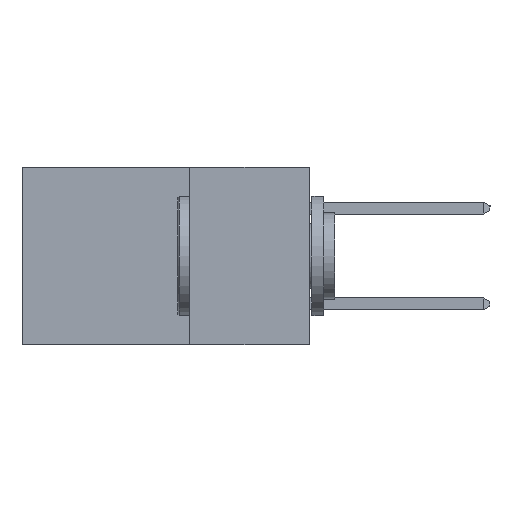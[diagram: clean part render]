
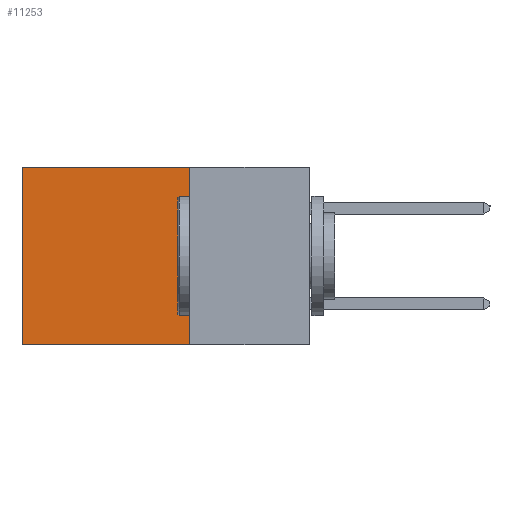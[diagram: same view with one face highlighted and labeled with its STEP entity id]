
A CAD part, left-side view. The second image highlights one B-rep face of the part: STEP entity #11253.
In plain terms, the highlighted planar face has unit normal (-1, 0, 0).
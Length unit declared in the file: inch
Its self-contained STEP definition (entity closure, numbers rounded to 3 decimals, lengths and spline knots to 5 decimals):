
#400 = CARTESIAN_POINT ( 'NONE',  ( 0.2875, 0.25, -0.37 ) ) ;
#543 = EDGE_CURVE ( 'NONE', #21170, #3944, #23759, .T. ) ;
#1645 = DIRECTION ( 'NONE',  ( 0., 0., -1. ) ) ;
#1817 = VECTOR ( 'NONE', #15721, 39.37008 ) ;
#2220 = VECTOR ( 'NONE', #1645, 39.37008 ) ;
#2248 = LINE ( 'NONE', #12837, #2220 ) ;
#3517 = ORIENTED_EDGE ( 'NONE', *, *, #543, .T. ) ;
#3944 = VERTEX_POINT ( 'NONE', #4181 ) ;
#3992 = ORIENTED_EDGE ( 'NONE', *, *, #23290, .F. ) ;
#4181 = CARTESIAN_POINT ( 'NONE',  ( 0.2875, 0.6, 0. ) ) ;
#4559 = DIRECTION ( 'NONE',  ( 0., 1., 0. ) ) ;
#8559 = AXIS2_PLACEMENT_3D ( 'NONE', #21134, #13468, #10036 ) ;
#9028 = LINE ( 'NONE', #400, #1817 ) ;
#9250 = DIRECTION ( 'NONE',  ( 0., 0., -1. ) ) ;
#10036 = DIRECTION ( 'NONE',  ( 0., 0., -1. ) ) ;
#10283 = VECTOR ( 'NONE', #9250, 39.37008 ) ;
#11253 = ADVANCED_FACE ( 'NONE', ( #19253 ), #17332, .F. ) ;
#11275 = VERTEX_POINT ( 'NONE', #15325 ) ;
#11772 = CARTESIAN_POINT ( 'NONE',  ( 0.2875, 0.25, 0. ) ) ;
#12328 = CARTESIAN_POINT ( 'NONE',  ( 0.2875, 0.25, 0. ) ) ;
#12645 = VERTEX_POINT ( 'NONE', #14042 ) ;
#12659 = ORIENTED_EDGE ( 'NONE', *, *, #13279, .F. ) ;
#12837 = CARTESIAN_POINT ( 'NONE',  ( 0.2875, 0.6, 0. ) ) ;
#13279 = EDGE_CURVE ( 'NONE', #12645, #11275, #9028, .T. ) ;
#13468 = DIRECTION ( 'NONE',  ( 1., 0., 0. ) ) ;
#13876 = ORIENTED_EDGE ( 'NONE', *, *, #22734, .T. ) ;
#14042 = CARTESIAN_POINT ( 'NONE',  ( 0.2875, 0.25, -0.37 ) ) ;
#14364 = LINE ( 'NONE', #12328, #10283 ) ;
#15325 = CARTESIAN_POINT ( 'NONE',  ( 0.2875, 0.6, -0.37 ) ) ;
#15721 = DIRECTION ( 'NONE',  ( 0., 1., 0. ) ) ;
#16295 = VECTOR ( 'NONE', #4559, 39.37008 ) ;
#17332 = PLANE ( 'NONE',  #8559 ) ;
#17521 = EDGE_LOOP ( 'NONE', ( #13876, #12659, #3992, #3517 ) ) ;
#18641 = CARTESIAN_POINT ( 'NONE',  ( 0.2875, 0.25, 0. ) ) ;
#19253 = FACE_OUTER_BOUND ( 'NONE', #17521, .T. ) ;
#21134 = CARTESIAN_POINT ( 'NONE',  ( 0.2875, 0.25, 0. ) ) ;
#21170 = VERTEX_POINT ( 'NONE', #18641 ) ;
#22734 = EDGE_CURVE ( 'NONE', #3944, #11275, #2248, .T. ) ;
#23290 = EDGE_CURVE ( 'NONE', #21170, #12645, #14364, .T. ) ;
#23759 = LINE ( 'NONE', #11772, #16295 ) ;
